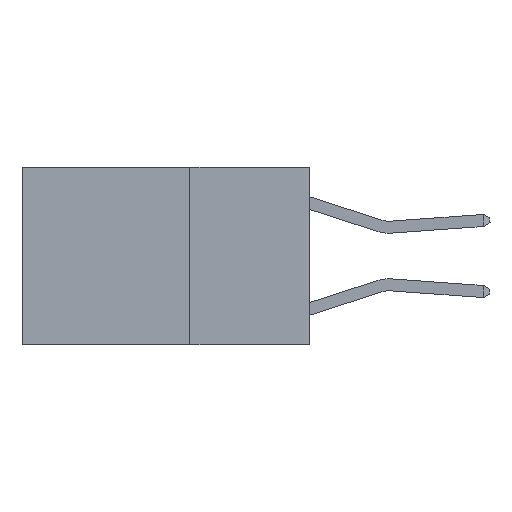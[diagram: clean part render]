
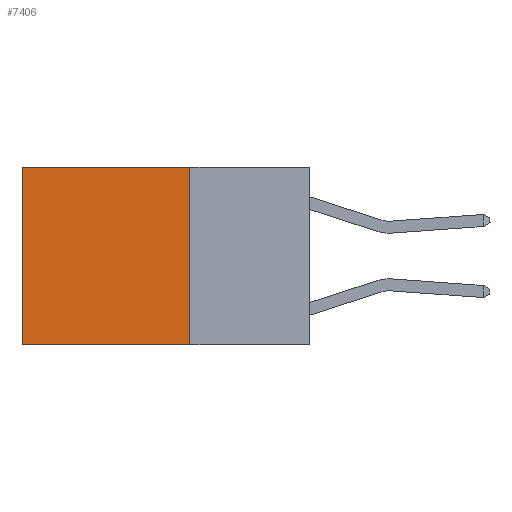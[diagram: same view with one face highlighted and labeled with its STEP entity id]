
A CAD part, left-side view. The second image highlights one B-rep face of the part: STEP entity #7406.
In plain terms, the highlighted planar face has unit normal (-1, 0, 0).
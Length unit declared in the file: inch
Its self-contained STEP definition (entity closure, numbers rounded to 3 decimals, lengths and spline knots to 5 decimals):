
#425 = CARTESIAN_POINT ( 'NONE',  ( 0.2625, 0.25, 0. ) ) ;
#692 = DIRECTION ( 'NONE',  ( 1., 0., 0. ) ) ;
#1179 = EDGE_LOOP ( 'NONE', ( #9767, #4227, #10123, #10788 ) ) ;
#1267 = DIRECTION ( 'NONE',  ( 0., 1., 0. ) ) ;
#1740 = DIRECTION ( 'NONE',  ( 0., 0., -1. ) ) ;
#2168 = LINE ( 'NONE', #11721, #12218 ) ;
#2652 = VERTEX_POINT ( 'NONE', #8707 ) ;
#2902 = EDGE_CURVE ( 'NONE', #2652, #4996, #15173, .T. ) ;
#4124 = EDGE_CURVE ( 'NONE', #12182, #12025, #15357, .T. ) ;
#4227 = ORIENTED_EDGE ( 'NONE', *, *, #2902, .F. ) ;
#4996 = VERTEX_POINT ( 'NONE', #11081 ) ;
#5461 = EDGE_CURVE ( 'NONE', #12025, #4996, #2168, .T. ) ;
#7175 = CARTESIAN_POINT ( 'NONE',  ( 0.2625, 0.25, 0. ) ) ;
#7406 = ADVANCED_FACE ( 'NONE', ( #12197 ), #16103, .F. ) ;
#8143 = VECTOR ( 'NONE', #16077, 39.37008 ) ;
#8707 = CARTESIAN_POINT ( 'NONE',  ( 0.2625, 0.25, -0.37 ) ) ;
#9201 = EDGE_CURVE ( 'NONE', #12182, #2652, #11939, .T. ) ;
#9767 = ORIENTED_EDGE ( 'NONE', *, *, #5461, .T. ) ;
#9926 = DIRECTION ( 'NONE',  ( 0., 0., -1. ) ) ;
#10123 = ORIENTED_EDGE ( 'NONE', *, *, #9201, .F. ) ;
#10788 = ORIENTED_EDGE ( 'NONE', *, *, #4124, .T. ) ;
#11081 = CARTESIAN_POINT ( 'NONE',  ( 0.2625, 0.6, -0.37 ) ) ;
#11557 = VECTOR ( 'NONE', #1740, 39.37008 ) ;
#11721 = CARTESIAN_POINT ( 'NONE',  ( 0.2625, 0.6, 0. ) ) ;
#11881 = VECTOR ( 'NONE', #1267, 39.37008 ) ;
#11939 = LINE ( 'NONE', #425, #11557 ) ;
#12025 = VERTEX_POINT ( 'NONE', #13976 ) ;
#12182 = VERTEX_POINT ( 'NONE', #14039 ) ;
#12197 = FACE_OUTER_BOUND ( 'NONE', #1179, .T. ) ;
#12218 = VECTOR ( 'NONE', #12893, 39.37008 ) ;
#12893 = DIRECTION ( 'NONE',  ( 0., 0., -1. ) ) ;
#13637 = CARTESIAN_POINT ( 'NONE',  ( 0.2625, 0.25, 0. ) ) ;
#13976 = CARTESIAN_POINT ( 'NONE',  ( 0.2625, 0.6, 0. ) ) ;
#14039 = CARTESIAN_POINT ( 'NONE',  ( 0.2625, 0.25, 0. ) ) ;
#15173 = LINE ( 'NONE', #15439, #11881 ) ;
#15357 = LINE ( 'NONE', #13637, #8143 ) ;
#15439 = CARTESIAN_POINT ( 'NONE',  ( 0.2625, 0.25, -0.37 ) ) ;
#15708 = AXIS2_PLACEMENT_3D ( 'NONE', #7175, #692, #9926 ) ;
#16077 = DIRECTION ( 'NONE',  ( 0., 1., 0. ) ) ;
#16103 = PLANE ( 'NONE',  #15708 ) ;
